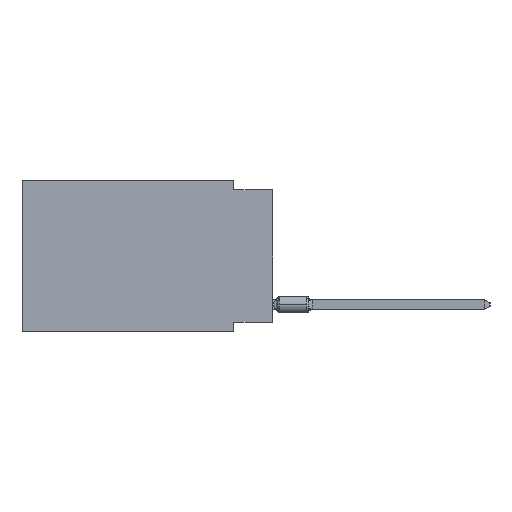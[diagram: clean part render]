
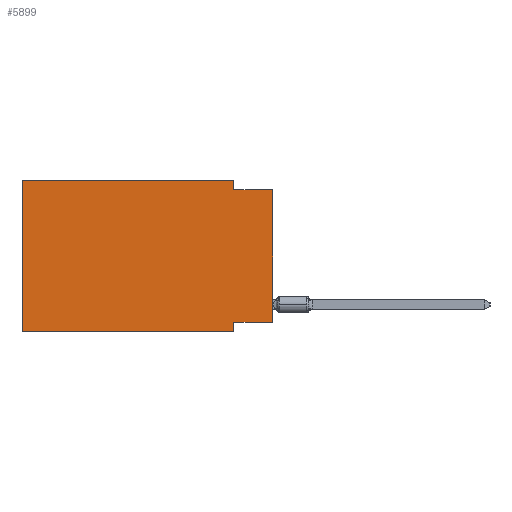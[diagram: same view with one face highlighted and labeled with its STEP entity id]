
A CAD part, left-side view. The second image highlights one B-rep face of the part: STEP entity #5899.
In plain terms, the highlighted planar face has unit normal (-1, 0, 0).
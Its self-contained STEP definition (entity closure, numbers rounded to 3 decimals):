
#1822 = CARTESIAN_POINT ( 'NONE',  ( 0., 16.383, 0. ) ) ;
#1905 = ORIENTED_EDGE ( 'NONE', *, *, #30154, .T. ) ;
#2169 = PLANE ( 'NONE',  #26708 ) ;
#2988 = DIRECTION ( 'NONE',  ( 0., 0., 1. ) ) ;
#3262 = VERTEX_POINT ( 'NONE', #14127 ) ;
#3465 = EDGE_LOOP ( 'NONE', ( #1905, #22723, #39513, #25741, #33957, #24493, #37011, #38453 ) ) ;
#5053 = DIRECTION ( 'NONE',  ( 0., 1., 0. ) ) ;
#5899 = ADVANCED_FACE ( 'NONE', ( #19208 ), #2169, .F. ) ;
#5986 = DIRECTION ( 'NONE',  ( 1., 0., 0. ) ) ;
#6346 = VECTOR ( 'NONE', #6619, 1000. ) ;
#6619 = DIRECTION ( 'NONE',  ( 0., -1., 0. ) ) ;
#8248 = VERTEX_POINT ( 'NONE', #1822 ) ;
#9388 = EDGE_CURVE ( 'NONE', #3262, #26260, #13351, .T. ) ;
#11236 = VECTOR ( 'NONE', #38733, 1000. ) ;
#11553 = VECTOR ( 'NONE', #5053, 1000. ) ;
#12080 = LINE ( 'NONE', #25771, #12445 ) ;
#12292 = VECTOR ( 'NONE', #2988, 1000. ) ;
#12359 = CARTESIAN_POINT ( 'NONE',  ( 0., 2.54, -9.271 ) ) ;
#12445 = VECTOR ( 'NONE', #44093, 1000. ) ;
#12970 = LINE ( 'NONE', #43432, #14960 ) ;
#13351 = LINE ( 'NONE', #40681, #6346 ) ;
#13638 = DIRECTION ( 'NONE',  ( 0., -1., 0. ) ) ;
#14127 = CARTESIAN_POINT ( 'NONE',  ( 0., 16.383, -9.906 ) ) ;
#14796 = VERTEX_POINT ( 'NONE', #26247 ) ;
#14960 = VECTOR ( 'NONE', #44308, 1000. ) ;
#15847 = CARTESIAN_POINT ( 'NONE',  ( 0., 16.383, 0. ) ) ;
#16994 = LINE ( 'NONE', #30667, #38932 ) ;
#17554 = VERTEX_POINT ( 'NONE', #37745 ) ;
#18449 = CARTESIAN_POINT ( 'NONE',  ( 0., 2.54, 0. ) ) ;
#18828 = LINE ( 'NONE', #38310, #24757 ) ;
#19208 = FACE_OUTER_BOUND ( 'NONE', #3465, .T. ) ;
#19687 = EDGE_CURVE ( 'NONE', #8248, #20388, #18828, .T. ) ;
#20388 = VERTEX_POINT ( 'NONE', #18449 ) ;
#22723 = ORIENTED_EDGE ( 'NONE', *, *, #34008, .F. ) ;
#22922 = EDGE_CURVE ( 'NONE', #3262, #8248, #29314, .T. ) ;
#23823 = LINE ( 'NONE', #37469, #12292 ) ;
#24493 = ORIENTED_EDGE ( 'NONE', *, *, #9388, .T. ) ;
#24757 = VECTOR ( 'NONE', #28690, 1000. ) ;
#25073 = EDGE_CURVE ( 'NONE', #37295, #26260, #12970, .T. ) ;
#25741 = ORIENTED_EDGE ( 'NONE', *, *, #19687, .F. ) ;
#25771 = CARTESIAN_POINT ( 'NONE',  ( 0., 2.54, 0. ) ) ;
#26247 = CARTESIAN_POINT ( 'NONE',  ( 0., 0., -0.635 ) ) ;
#26260 = VERTEX_POINT ( 'NONE', #35625 ) ;
#26708 = AXIS2_PLACEMENT_3D ( 'NONE', #15847, #5986, #29514 ) ;
#28690 = DIRECTION ( 'NONE',  ( 0., -1., 0. ) ) ;
#28819 = LINE ( 'NONE', #32183, #11553 ) ;
#29314 = LINE ( 'NONE', #42966, #11236 ) ;
#29502 = EDGE_CURVE ( 'NONE', #32177, #37295, #28819, .T. ) ;
#29514 = DIRECTION ( 'NONE',  ( 0., 0., -1. ) ) ;
#30154 = EDGE_CURVE ( 'NONE', #32177, #14796, #23823, .T. ) ;
#30667 = CARTESIAN_POINT ( 'NONE',  ( 0., 0., -0.635 ) ) ;
#32177 = VERTEX_POINT ( 'NONE', #37147 ) ;
#32183 = CARTESIAN_POINT ( 'NONE',  ( 0., 0., -9.271 ) ) ;
#33785 = EDGE_CURVE ( 'NONE', #20388, #17554, #12080, .T. ) ;
#33957 = ORIENTED_EDGE ( 'NONE', *, *, #22922, .F. ) ;
#34008 = EDGE_CURVE ( 'NONE', #17554, #14796, #16994, .T. ) ;
#35625 = CARTESIAN_POINT ( 'NONE',  ( 0., 2.54, -9.906 ) ) ;
#37011 = ORIENTED_EDGE ( 'NONE', *, *, #25073, .F. ) ;
#37147 = CARTESIAN_POINT ( 'NONE',  ( 0., 0., -9.271 ) ) ;
#37295 = VERTEX_POINT ( 'NONE', #12359 ) ;
#37469 = CARTESIAN_POINT ( 'NONE',  ( 0., 0., 0. ) ) ;
#37745 = CARTESIAN_POINT ( 'NONE',  ( 0., 2.54, -0.635 ) ) ;
#38310 = CARTESIAN_POINT ( 'NONE',  ( 0., 16.383, 0. ) ) ;
#38453 = ORIENTED_EDGE ( 'NONE', *, *, #29502, .F. ) ;
#38733 = DIRECTION ( 'NONE',  ( 0., 0., 1. ) ) ;
#38932 = VECTOR ( 'NONE', #13638, 1000. ) ;
#39513 = ORIENTED_EDGE ( 'NONE', *, *, #33785, .F. ) ;
#40681 = CARTESIAN_POINT ( 'NONE',  ( 0., 16.383, -9.906 ) ) ;
#42966 = CARTESIAN_POINT ( 'NONE',  ( 0., 16.383, 0. ) ) ;
#43432 = CARTESIAN_POINT ( 'NONE',  ( 0., 2.54, -9.906 ) ) ;
#44093 = DIRECTION ( 'NONE',  ( 0., 0., -1. ) ) ;
#44308 = DIRECTION ( 'NONE',  ( 0., 0., -1. ) ) ;
